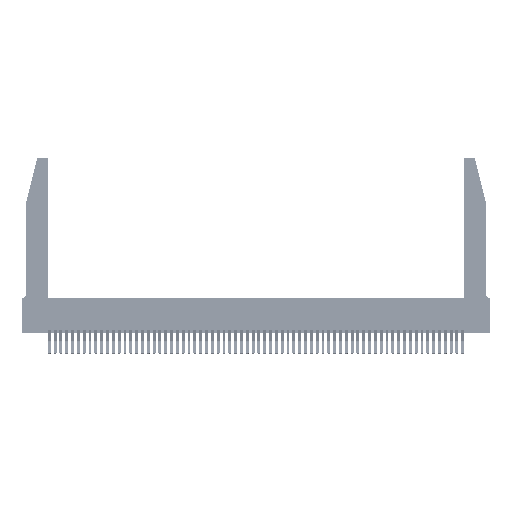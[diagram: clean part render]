
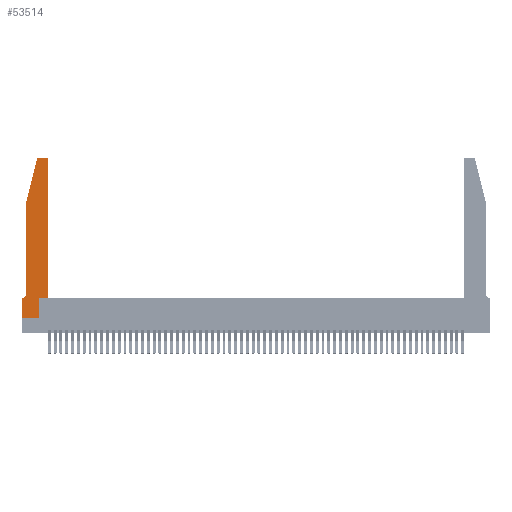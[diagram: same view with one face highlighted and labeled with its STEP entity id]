
A CAD part, top view. The second image highlights one B-rep face of the part: STEP entity #53514.
In plain terms, the highlighted planar face has unit normal (0, 0, 1).
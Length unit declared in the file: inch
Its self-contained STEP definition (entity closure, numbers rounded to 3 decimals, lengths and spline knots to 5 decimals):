
#640 = ORIENTED_EDGE ( 'NONE', *, *, #33612, .T. ) ;
#3270 = EDGE_CURVE ( 'NONE', #32792, #57231, #48510, .T. ) ;
#3773 = DIRECTION ( 'NONE',  ( -1., 0., 0. ) ) ;
#4110 = VECTOR ( 'NONE', #22556, 39.37008 ) ;
#4874 = CARTESIAN_POINT ( 'NONE',  ( 0.0755, 2., 0.37 ) ) ;
#6070 = CARTESIAN_POINT ( 'NONE',  ( 0.0755, 0.35, 0.37 ) ) ;
#6259 = DIRECTION ( 'NONE',  ( 0., 0., 1. ) ) ;
#6744 = LINE ( 'NONE', #6070, #52295 ) ;
#6872 = ORIENTED_EDGE ( 'NONE', *, *, #38305, .T. ) ;
#7153 = EDGE_CURVE ( 'NONE', #15173, #22044, #6744, .T. ) ;
#7160 = EDGE_CURVE ( 'NONE', #17910, #48291, #19886, .T. ) ;
#9472 = ORIENTED_EDGE ( 'NONE', *, *, #49144, .T. ) ;
#9846 = LINE ( 'NONE', #12421, #53991 ) ;
#11211 = DIRECTION ( 'NONE',  ( 0., -1., 0. ) ) ;
#11382 = VERTEX_POINT ( 'NONE', #20711 ) ;
#11654 = DIRECTION ( 'NONE',  ( 0., 1., 0. ) ) ;
#12421 = CARTESIAN_POINT ( 'NONE',  ( 0.0755, 2., 0.37 ) ) ;
#12774 = EDGE_LOOP ( 'NONE', ( #9472, #22233, #53182, #45379, #33313, #55152, #37714, #31085, #6872, #42971, #640, #18955 ) ) ;
#12949 = VERTEX_POINT ( 'NONE', #17540 ) ;
#13344 = CARTESIAN_POINT ( 'NONE',  ( 0., 0., 0.37 ) ) ;
#15173 = VERTEX_POINT ( 'NONE', #55127 ) ;
#15260 = CARTESIAN_POINT ( 'NONE',  ( 0.4205, 2.72, 0.37 ) ) ;
#17540 = CARTESIAN_POINT ( 'NONE',  ( 0.2865, 0.35, 0.37 ) ) ;
#17750 = VECTOR ( 'NONE', #40252, 39.37008 ) ;
#17910 = VERTEX_POINT ( 'NONE', #35478 ) ;
#17988 = EDGE_CURVE ( 'NONE', #48291, #28822, #52948, .T. ) ;
#18112 = CARTESIAN_POINT ( 'NONE',  ( 0.4505, 0.35, 0.37 ) ) ;
#18955 = ORIENTED_EDGE ( 'NONE', *, *, #3270, .T. ) ;
#19677 = DIRECTION ( 'NONE',  ( 1., 0., 0. ) ) ;
#19886 = CIRCLE ( 'NONE', #50866, 0.03 ) ;
#20491 = VECTOR ( 'NONE', #35578, 39.37008 ) ;
#20711 = CARTESIAN_POINT ( 'NONE',  ( 0.0755, 0.42, 0.37 ) ) ;
#21443 = CARTESIAN_POINT ( 'NONE',  ( 0.2605, 2.75, 0.37 ) ) ;
#21464 = DIRECTION ( 'NONE',  ( 0., 0., 1. ) ) ;
#22044 = VERTEX_POINT ( 'NONE', #42708 ) ;
#22233 = ORIENTED_EDGE ( 'NONE', *, *, #7160, .T. ) ;
#22556 = DIRECTION ( 'NONE',  ( 1., 0., 0. ) ) ;
#23127 = CIRCLE ( 'NONE', #52985, 0.07 ) ;
#23176 = CARTESIAN_POINT ( 'NONE',  ( 0.25487, 2.72718, 0.37 ) ) ;
#23762 = LINE ( 'NONE', #21443, #34185 ) ;
#25112 = DIRECTION ( 'NONE',  ( 0., 0., -1. ) ) ;
#25751 = DIRECTION ( 'NONE',  ( 0., -1., 0. ) ) ;
#25759 = LINE ( 'NONE', #29859, #47788 ) ;
#26387 = AXIS2_PLACEMENT_3D ( 'NONE', #15260, #46079, #19677 ) ;
#28822 = VERTEX_POINT ( 'NONE', #29443 ) ;
#29421 = CARTESIAN_POINT ( 'NONE',  ( 0.4505, 0.35, 0.37 ) ) ;
#29443 = CARTESIAN_POINT ( 'NONE',  ( 0.0755, 2., 0.37 ) ) ;
#29527 = EDGE_CURVE ( 'NONE', #11382, #15173, #23127, .T. ) ;
#29859 = CARTESIAN_POINT ( 'NONE',  ( 0.2865, 0.35, 0.37 ) ) ;
#30921 = VERTEX_POINT ( 'NONE', #34090 ) ;
#30970 = EDGE_CURVE ( 'NONE', #28822, #11382, #9846, .T. ) ;
#31085 = ORIENTED_EDGE ( 'NONE', *, *, #46119, .T. ) ;
#32281 = LINE ( 'NONE', #13344, #20491 ) ;
#32608 = DIRECTION ( 'NONE',  ( -1., 0., 0. ) ) ;
#32792 = VERTEX_POINT ( 'NONE', #47693 ) ;
#32803 = CARTESIAN_POINT ( 'NONE',  ( 0.284, 2.72, 0.37 ) ) ;
#33313 = ORIENTED_EDGE ( 'NONE', *, *, #29527, .T. ) ;
#33498 = VECTOR ( 'NONE', #11211, 39.37008 ) ;
#33612 = EDGE_CURVE ( 'NONE', #43453, #32792, #52420, .T. ) ;
#34090 = CARTESIAN_POINT ( 'NONE',  ( 0.2865, 0., 0.37 ) ) ;
#34185 = VECTOR ( 'NONE', #3773, 39.37008 ) ;
#34320 = DIRECTION ( 'NONE',  ( 0., 1., 0. ) ) ;
#35478 = CARTESIAN_POINT ( 'NONE',  ( 0.284, 2.75, 0.37 ) ) ;
#35578 = DIRECTION ( 'NONE',  ( 1., 0., 0. ) ) ;
#37202 = DIRECTION ( 'NONE',  ( 1., 0., 0. ) ) ;
#37452 = EDGE_CURVE ( 'NONE', #22044, #46949, #37614, .T. ) ;
#37614 = LINE ( 'NONE', #42067, #33498 ) ;
#37714 = ORIENTED_EDGE ( 'NONE', *, *, #37452, .T. ) ;
#38305 = EDGE_CURVE ( 'NONE', #30921, #12949, #25759, .T. ) ;
#39333 = VECTOR ( 'NONE', #11654, 39.37008 ) ;
#39407 = LINE ( 'NONE', #18112, #4110 ) ;
#40252 = DIRECTION ( 'NONE',  ( -0.239, -0.971, 0. ) ) ;
#42067 = CARTESIAN_POINT ( 'NONE',  ( 0., 0., 0.37 ) ) ;
#42708 = CARTESIAN_POINT ( 'NONE',  ( 0., 0.35, 0.37 ) ) ;
#42971 = ORIENTED_EDGE ( 'NONE', *, *, #43739, .T. ) ;
#43421 = PLANE ( 'NONE',  #50019 ) ;
#43453 = VERTEX_POINT ( 'NONE', #50555 ) ;
#43739 = EDGE_CURVE ( 'NONE', #12949, #43453, #39407, .T. ) ;
#45220 = CARTESIAN_POINT ( 'NONE',  ( 0.4205, 2.75, 0.37 ) ) ;
#45379 = ORIENTED_EDGE ( 'NONE', *, *, #30970, .T. ) ;
#46079 = DIRECTION ( 'NONE',  ( 0., 0., 1. ) ) ;
#46119 = EDGE_CURVE ( 'NONE', #46949, #30921, #32281, .T. ) ;
#46949 = VERTEX_POINT ( 'NONE', #49917 ) ;
#47693 = CARTESIAN_POINT ( 'NONE',  ( 0.4505, 2.72, 0.37 ) ) ;
#47788 = VECTOR ( 'NONE', #34320, 39.37008 ) ;
#47847 = CARTESIAN_POINT ( 'NONE',  ( 0., 0.35, 0.37 ) ) ;
#48291 = VERTEX_POINT ( 'NONE', #23176 ) ;
#48510 = CIRCLE ( 'NONE', #26387, 0.03 ) ;
#49144 = EDGE_CURVE ( 'NONE', #57231, #17910, #23762, .T. ) ;
#49917 = CARTESIAN_POINT ( 'NONE',  ( 0., 0., 0.37 ) ) ;
#50019 = AXIS2_PLACEMENT_3D ( 'NONE', #47847, #21464, #52298 ) ;
#50555 = CARTESIAN_POINT ( 'NONE',  ( 0.4505, 0.35, 0.37 ) ) ;
#50866 = AXIS2_PLACEMENT_3D ( 'NONE', #32803, #6259, #37202 ) ;
#51494 = CARTESIAN_POINT ( 'NONE',  ( 0.0055, 0.42, 0.37 ) ) ;
#52180 = FACE_OUTER_BOUND ( 'NONE', #12774, .T. ) ;
#52295 = VECTOR ( 'NONE', #32608, 39.37008 ) ;
#52298 = DIRECTION ( 'NONE',  ( 1., 0., 0. ) ) ;
#52420 = LINE ( 'NONE', #29421, #39333 ) ;
#52948 = LINE ( 'NONE', #4874, #17750 ) ;
#52985 = AXIS2_PLACEMENT_3D ( 'NONE', #51494, #25112, #55932 ) ;
#53182 = ORIENTED_EDGE ( 'NONE', *, *, #17988, .T. ) ;
#53514 = ADVANCED_FACE ( 'NONE', ( #52180 ), #43421, .T. ) ;
#53991 = VECTOR ( 'NONE', #25751, 39.37008 ) ;
#55127 = CARTESIAN_POINT ( 'NONE',  ( 0.0055, 0.35, 0.37 ) ) ;
#55152 = ORIENTED_EDGE ( 'NONE', *, *, #7153, .T. ) ;
#55932 = DIRECTION ( 'NONE',  ( -1., 0., 0. ) ) ;
#57231 = VERTEX_POINT ( 'NONE', #45220 ) ;
